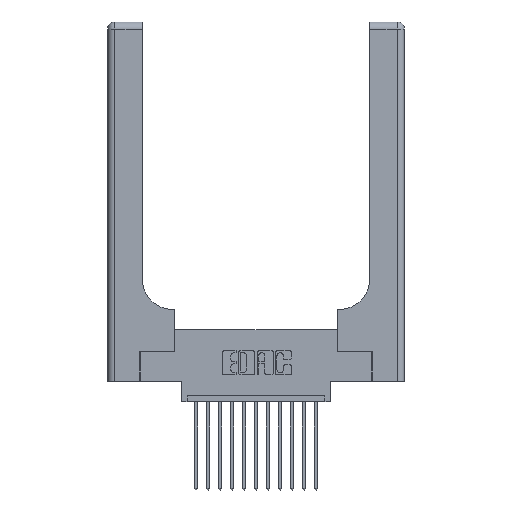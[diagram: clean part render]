
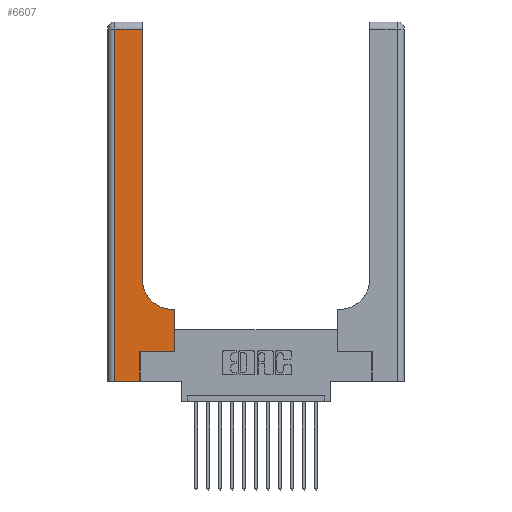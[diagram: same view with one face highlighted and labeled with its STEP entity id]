
A CAD part, top view. The second image highlights one B-rep face of the part: STEP entity #6607.
In plain terms, the highlighted planar face has unit normal (0, 0, 1).
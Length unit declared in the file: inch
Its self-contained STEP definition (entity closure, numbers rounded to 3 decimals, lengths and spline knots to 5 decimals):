
#163 = CARTESIAN_POINT ( 'NONE',  ( 0.06, 2.94, 0.37 ) ) ;
#565 = VERTEX_POINT ( 'NONE', #13423 ) ;
#1059 = EDGE_CURVE ( 'NONE', #2668, #2970, #4531, .T. ) ;
#1318 = EDGE_CURVE ( 'NONE', #14735, #11284, #13333, .T. ) ;
#1552 = ORIENTED_EDGE ( 'NONE', *, *, #6407, .T. ) ;
#1900 = EDGE_CURVE ( 'NONE', #15197, #7851, #12653, .T. ) ;
#2143 = EDGE_CURVE ( 'NONE', #12341, #15197, #17810, .T. ) ;
#2264 = CARTESIAN_POINT ( 'NONE',  ( 0.5415, 0.6, 0.37 ) ) ;
#2303 = CARTESIAN_POINT ( 'NONE',  ( 0.5415, 0.85, 0.37 ) ) ;
#2668 = VERTEX_POINT ( 'NONE', #11784 ) ;
#2963 = DIRECTION ( 'NONE',  ( 0., 0., -1. ) ) ;
#2970 = VERTEX_POINT ( 'NONE', #2264 ) ;
#3045 = VECTOR ( 'NONE', #7933, 39.37008 ) ;
#3303 = FACE_OUTER_BOUND ( 'NONE', #14675, .T. ) ;
#3423 = VECTOR ( 'NONE', #11840, 39.37008 ) ;
#4531 = LINE ( 'NONE', #7766, #3045 ) ;
#4662 = DIRECTION ( 'NONE',  ( 1., 0., 0. ) ) ;
#5013 = VECTOR ( 'NONE', #9162, 39.37008 ) ;
#5117 = CARTESIAN_POINT ( 'NONE',  ( 0.5585, 0.25, 0.37 ) ) ;
#5228 = DIRECTION ( 'NONE',  ( 0., 0., -1. ) ) ;
#5623 = CARTESIAN_POINT ( 'NONE',  ( 0.2915, 3., 0.37 ) ) ;
#5644 = PLANE ( 'NONE',  #8914 ) ;
#5695 = ORIENTED_EDGE ( 'NONE', *, *, #1900, .T. ) ;
#5950 = AXIS2_PLACEMENT_3D ( 'NONE', #2303, #5228, #11886 ) ;
#6232 = CARTESIAN_POINT ( 'NONE',  ( 0., 2.94, 0.37 ) ) ;
#6407 = EDGE_CURVE ( 'NONE', #7851, #14735, #7154, .T. ) ;
#6607 = ADVANCED_FACE ( 'NONE', ( #3303 ), #5644, .F. ) ;
#6657 = LINE ( 'NONE', #5623, #14847 ) ;
#6852 = CARTESIAN_POINT ( 'NONE',  ( 0.06, 3., 0.37 ) ) ;
#6867 = CARTESIAN_POINT ( 'NONE',  ( 0.269, 0., 0.37 ) ) ;
#6886 = EDGE_CURVE ( 'NONE', #565, #12341, #11003, .T. ) ;
#7044 = CARTESIAN_POINT ( 'NONE',  ( 0., 3., 0.37 ) ) ;
#7154 = LINE ( 'NONE', #6867, #9286 ) ;
#7740 = VECTOR ( 'NONE', #15344, 39.37008 ) ;
#7766 = CARTESIAN_POINT ( 'NONE',  ( 0.2915, 0.6, 0.37 ) ) ;
#7851 = VERTEX_POINT ( 'NONE', #7896 ) ;
#7896 = CARTESIAN_POINT ( 'NONE',  ( 0.269, 0., 0.37 ) ) ;
#7933 = DIRECTION ( 'NONE',  ( -1., 0., 0. ) ) ;
#8110 = ORIENTED_EDGE ( 'NONE', *, *, #12937, .T. ) ;
#8633 = CARTESIAN_POINT ( 'NONE',  ( 0.269, 0.25, 0.37 ) ) ;
#8661 = LINE ( 'NONE', #10618, #5013 ) ;
#8914 = AXIS2_PLACEMENT_3D ( 'NONE', #7044, #2963, #13952 ) ;
#9162 = DIRECTION ( 'NONE',  ( 0., 1., 0. ) ) ;
#9286 = VECTOR ( 'NONE', #10987, 39.37008 ) ;
#9685 = DIRECTION ( 'NONE',  ( 0., 1., 0. ) ) ;
#10139 = ORIENTED_EDGE ( 'NONE', *, *, #6886, .T. ) ;
#10587 = ORIENTED_EDGE ( 'NONE', *, *, #2143, .T. ) ;
#10618 = CARTESIAN_POINT ( 'NONE',  ( 0.5585, 0.25, 0.37 ) ) ;
#10687 = CARTESIAN_POINT ( 'NONE',  ( 0., 0., 0.37 ) ) ;
#10768 = ORIENTED_EDGE ( 'NONE', *, *, #14341, .T. ) ;
#10987 = DIRECTION ( 'NONE',  ( 0., 1., 0. ) ) ;
#11003 = LINE ( 'NONE', #6232, #12728 ) ;
#11284 = VERTEX_POINT ( 'NONE', #5117 ) ;
#11487 = ORIENTED_EDGE ( 'NONE', *, *, #1318, .T. ) ;
#11784 = CARTESIAN_POINT ( 'NONE',  ( 0.5585, 0.6, 0.37 ) ) ;
#11840 = DIRECTION ( 'NONE',  ( 1., 0., 0. ) ) ;
#11886 = DIRECTION ( 'NONE',  ( 1., 0., 0. ) ) ;
#12332 = ORIENTED_EDGE ( 'NONE', *, *, #1059, .T. ) ;
#12341 = VERTEX_POINT ( 'NONE', #163 ) ;
#12653 = LINE ( 'NONE', #10687, #3423 ) ;
#12728 = VECTOR ( 'NONE', #14298, 39.37008 ) ;
#12937 = EDGE_CURVE ( 'NONE', #2970, #15730, #16456, .T. ) ;
#13333 = LINE ( 'NONE', #8633, #17423 ) ;
#13423 = CARTESIAN_POINT ( 'NONE',  ( 0.2915, 2.94, 0.37 ) ) ;
#13952 = DIRECTION ( 'NONE',  ( -1., 0., 0. ) ) ;
#14233 = CARTESIAN_POINT ( 'NONE',  ( 0.269, 0.25, 0.37 ) ) ;
#14298 = DIRECTION ( 'NONE',  ( -1., 0., 0. ) ) ;
#14341 = EDGE_CURVE ( 'NONE', #11284, #2668, #8661, .T. ) ;
#14572 = CARTESIAN_POINT ( 'NONE',  ( 0.06, 0., 0.37 ) ) ;
#14675 = EDGE_LOOP ( 'NONE', ( #17136, #10139, #10587, #5695, #1552, #11487, #10768, #12332, #8110 ) ) ;
#14735 = VERTEX_POINT ( 'NONE', #14233 ) ;
#14847 = VECTOR ( 'NONE', #9685, 39.37008 ) ;
#15197 = VERTEX_POINT ( 'NONE', #14572 ) ;
#15344 = DIRECTION ( 'NONE',  ( 0., -1., 0. ) ) ;
#15730 = VERTEX_POINT ( 'NONE', #16731 ) ;
#16456 = CIRCLE ( 'NONE', #5950, 0.25 ) ;
#16731 = CARTESIAN_POINT ( 'NONE',  ( 0.2915, 0.85, 0.37 ) ) ;
#17136 = ORIENTED_EDGE ( 'NONE', *, *, #17440, .T. ) ;
#17423 = VECTOR ( 'NONE', #4662, 39.37008 ) ;
#17440 = EDGE_CURVE ( 'NONE', #15730, #565, #6657, .T. ) ;
#17810 = LINE ( 'NONE', #6852, #7740 ) ;
